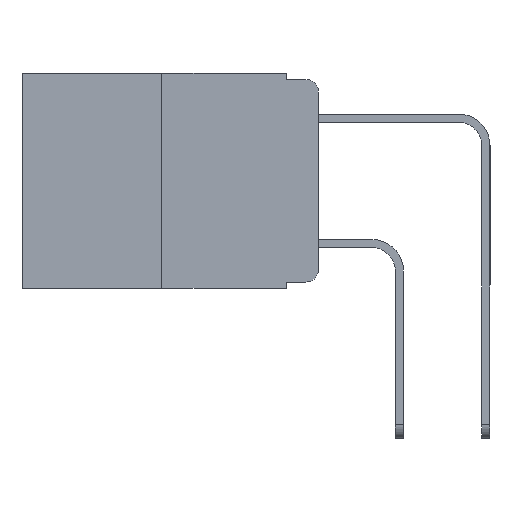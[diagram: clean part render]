
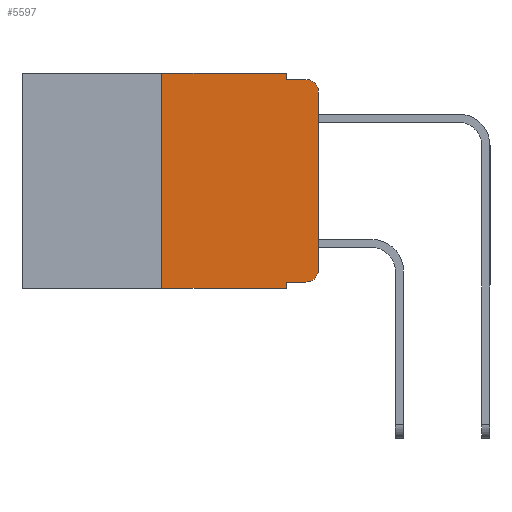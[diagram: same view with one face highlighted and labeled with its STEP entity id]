
A CAD part, left-side view. The second image highlights one B-rep face of the part: STEP entity #5597.
In plain terms, the highlighted planar face has unit normal (-1, 0, 0).
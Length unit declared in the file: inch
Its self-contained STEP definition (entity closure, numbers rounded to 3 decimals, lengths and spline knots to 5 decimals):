
#281 = VECTOR ( 'NONE', #1242, 39.37008 ) ;
#417 = CARTESIAN_POINT ( 'NONE',  ( 0., 0.051, -0.343 ) ) ;
#587 = EDGE_CURVE ( 'NONE', #10274, #13553, #3134, .T. ) ;
#858 = ORIENTED_EDGE ( 'NONE', *, *, #587, .T. ) ;
#867 = CARTESIAN_POINT ( 'NONE',  ( 0., 0., 0. ) ) ;
#868 = EDGE_CURVE ( 'NONE', #6818, #10274, #8876, .T. ) ;
#930 = VECTOR ( 'NONE', #9667, 39.37008 ) ;
#1242 = DIRECTION ( 'NONE',  ( 0., 0., -1. ) ) ;
#1559 = VERTEX_POINT ( 'NONE', #2087 ) ;
#1735 = CIRCLE ( 'NONE', #3584, 0.02 ) ;
#2087 = CARTESIAN_POINT ( 'NONE',  ( 0., 0.051, -0.01 ) ) ;
#2420 = VECTOR ( 'NONE', #17325, 39.37008 ) ;
#2573 = VERTEX_POINT ( 'NONE', #3667 ) ;
#2623 = PLANE ( 'NONE',  #8371 ) ;
#2771 = CARTESIAN_POINT ( 'NONE',  ( 0., 0.051, 0. ) ) ;
#3134 = CIRCLE ( 'NONE', #6940, 0.02 ) ;
#3584 = AXIS2_PLACEMENT_3D ( 'NONE', #12917, #4865, #14239 ) ;
#3667 = CARTESIAN_POINT ( 'NONE',  ( 0., 0.02, -0.01 ) ) ;
#3952 = DIRECTION ( 'NONE',  ( 0., 0., -1. ) ) ;
#4152 = DIRECTION ( 'NONE',  ( 0., 0., -1. ) ) ;
#4583 = EDGE_CURVE ( 'NONE', #6818, #15363, #11544, .T. ) ;
#4700 = VECTOR ( 'NONE', #6263, 39.37008 ) ;
#4805 = ORIENTED_EDGE ( 'NONE', *, *, #17331, .T. ) ;
#4865 = DIRECTION ( 'NONE',  ( -1., 0., 0. ) ) ;
#4927 = CARTESIAN_POINT ( 'NONE',  ( 0., 0.051, -0.333 ) ) ;
#5286 = CARTESIAN_POINT ( 'NONE',  ( 0., 0.473, 0. ) ) ;
#5428 = VECTOR ( 'NONE', #4152, 39.37008 ) ;
#5482 = ORIENTED_EDGE ( 'NONE', *, *, #5653, .F. ) ;
#5558 = DIRECTION ( 'NONE',  ( -1., 0., 0. ) ) ;
#5597 = ADVANCED_FACE ( 'NONE', ( #13983 ), #2623, .F. ) ;
#5653 = EDGE_CURVE ( 'NONE', #7644, #16479, #16598, .T. ) ;
#5853 = CARTESIAN_POINT ( 'NONE',  ( 0., 0.02, -0.313 ) ) ;
#5866 = ORIENTED_EDGE ( 'NONE', *, *, #10339, .F. ) ;
#6056 = ORIENTED_EDGE ( 'NONE', *, *, #10950, .F. ) ;
#6213 = ORIENTED_EDGE ( 'NONE', *, *, #4583, .F. ) ;
#6263 = DIRECTION ( 'NONE',  ( 0., -1., 0. ) ) ;
#6377 = ORIENTED_EDGE ( 'NONE', *, *, #6636, .T. ) ;
#6636 = EDGE_CURVE ( 'NONE', #17077, #15363, #14951, .T. ) ;
#6733 = ORIENTED_EDGE ( 'NONE', *, *, #868, .T. ) ;
#6818 = VERTEX_POINT ( 'NONE', #10631 ) ;
#6940 = AXIS2_PLACEMENT_3D ( 'NONE', #5853, #5558, #9142 ) ;
#6983 = CARTESIAN_POINT ( 'NONE',  ( 0., 0.051, 0. ) ) ;
#7096 = CARTESIAN_POINT ( 'NONE',  ( 0., 0.25, -0.343 ) ) ;
#7305 = EDGE_CURVE ( 'NONE', #12079, #2573, #1735, .T. ) ;
#7354 = EDGE_CURVE ( 'NONE', #17077, #7644, #14726, .T. ) ;
#7644 = VERTEX_POINT ( 'NONE', #8325 ) ;
#7685 = CARTESIAN_POINT ( 'NONE',  ( 0., 0.25, 0. ) ) ;
#7865 = ORIENTED_EDGE ( 'NONE', *, *, #7354, .F. ) ;
#8325 = CARTESIAN_POINT ( 'NONE',  ( 0., 0.25, 0. ) ) ;
#8327 = CARTESIAN_POINT ( 'NONE',  ( 0., 0.051, -0.01 ) ) ;
#8371 = AXIS2_PLACEMENT_3D ( 'NONE', #5286, #12030, #3952 ) ;
#8876 = LINE ( 'NONE', #4927, #15466 ) ;
#9142 = DIRECTION ( 'NONE',  ( 0., 0., -1. ) ) ;
#9308 = ORIENTED_EDGE ( 'NONE', *, *, #7305, .T. ) ;
#9428 = VECTOR ( 'NONE', #13034, 39.37008 ) ;
#9493 = CARTESIAN_POINT ( 'NONE',  ( 0., 0.473, 0. ) ) ;
#9667 = DIRECTION ( 'NONE',  ( 0., -1., 0. ) ) ;
#9854 = LINE ( 'NONE', #867, #9428 ) ;
#10274 = VERTEX_POINT ( 'NONE', #13505 ) ;
#10339 = EDGE_CURVE ( 'NONE', #1559, #2573, #12126, .T. ) ;
#10631 = CARTESIAN_POINT ( 'NONE',  ( 0., 0.051, -0.333 ) ) ;
#10732 = CARTESIAN_POINT ( 'NONE',  ( 0., 0.051, 0. ) ) ;
#10950 = EDGE_CURVE ( 'NONE', #16479, #1559, #12559, .T. ) ;
#11239 = VECTOR ( 'NONE', #16876, 39.37008 ) ;
#11544 = LINE ( 'NONE', #10732, #281 ) ;
#12030 = DIRECTION ( 'NONE',  ( 1., 0., 0. ) ) ;
#12079 = VERTEX_POINT ( 'NONE', #17113 ) ;
#12126 = LINE ( 'NONE', #8327, #930 ) ;
#12559 = LINE ( 'NONE', #2771, #5428 ) ;
#12711 = CARTESIAN_POINT ( 'NONE',  ( 0., 0., -0.313 ) ) ;
#12917 = CARTESIAN_POINT ( 'NONE',  ( 0., 0.02, -0.03 ) ) ;
#13034 = DIRECTION ( 'NONE',  ( 0., 0., 1. ) ) ;
#13505 = CARTESIAN_POINT ( 'NONE',  ( 0., 0.02, -0.333 ) ) ;
#13553 = VERTEX_POINT ( 'NONE', #12711 ) ;
#13983 = FACE_OUTER_BOUND ( 'NONE', #15121, .T. ) ;
#14239 = DIRECTION ( 'NONE',  ( 0., 0., -1. ) ) ;
#14260 = CARTESIAN_POINT ( 'NONE',  ( 0., 0.473, -0.343 ) ) ;
#14726 = LINE ( 'NONE', #7685, #11239 ) ;
#14951 = LINE ( 'NONE', #14260, #4700 ) ;
#15121 = EDGE_LOOP ( 'NONE', ( #4805, #9308, #5866, #6056, #5482, #7865, #6377, #6213, #6733, #858 ) ) ;
#15363 = VERTEX_POINT ( 'NONE', #417 ) ;
#15466 = VECTOR ( 'NONE', #16605, 39.37008 ) ;
#16479 = VERTEX_POINT ( 'NONE', #6983 ) ;
#16598 = LINE ( 'NONE', #9493, #2420 ) ;
#16605 = DIRECTION ( 'NONE',  ( 0., -1., 0. ) ) ;
#16876 = DIRECTION ( 'NONE',  ( 0., 0., 1. ) ) ;
#17077 = VERTEX_POINT ( 'NONE', #7096 ) ;
#17113 = CARTESIAN_POINT ( 'NONE',  ( 0., 0., -0.03 ) ) ;
#17325 = DIRECTION ( 'NONE',  ( 0., -1., 0. ) ) ;
#17331 = EDGE_CURVE ( 'NONE', #13553, #12079, #9854, .T. ) ;
